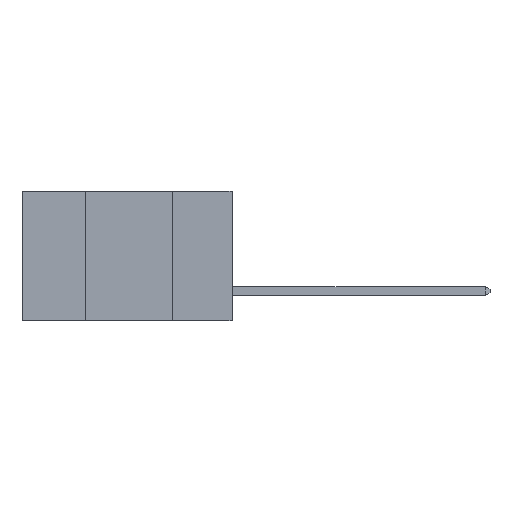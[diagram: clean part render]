
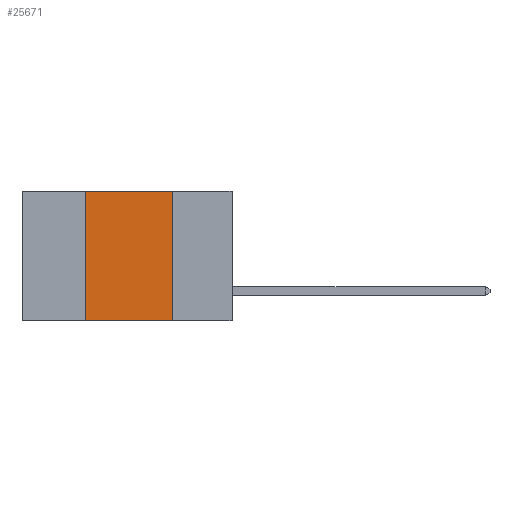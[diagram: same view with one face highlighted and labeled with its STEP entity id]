
A CAD part, left-side view. The second image highlights one B-rep face of the part: STEP entity #25671.
In plain terms, the highlighted planar face has unit normal (-1, 0, 0).
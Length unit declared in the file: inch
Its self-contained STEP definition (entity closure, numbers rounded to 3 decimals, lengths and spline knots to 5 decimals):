
#532 = VERTEX_POINT ( 'NONE', #34800 ) ;
#2224 = ORIENTED_EDGE ( 'NONE', *, *, #3149, .F. ) ;
#2685 = VERTEX_POINT ( 'NONE', #16816 ) ;
#2779 = DIRECTION ( 'NONE',  ( 0., 0., -1. ) ) ;
#3076 = LINE ( 'NONE', #16476, #35487 ) ;
#3149 = EDGE_CURVE ( 'NONE', #21279, #20346, #15940, .T. ) ;
#3304 = DIRECTION ( 'NONE',  ( 0., -1., 0. ) ) ;
#5337 = ORIENTED_EDGE ( 'NONE', *, *, #33064, .F. ) ;
#8743 = CARTESIAN_POINT ( 'NONE',  ( 0., 0.42, 0. ) ) ;
#14089 = ORIENTED_EDGE ( 'NONE', *, *, #38648, .F. ) ;
#15940 = LINE ( 'NONE', #41463, #35038 ) ;
#16476 = CARTESIAN_POINT ( 'NONE',  ( 0., 0.6, -0.37 ) ) ;
#16816 = CARTESIAN_POINT ( 'NONE',  ( 0., 0.42, 0. ) ) ;
#17154 = ORIENTED_EDGE ( 'NONE', *, *, #32216, .T. ) ;
#20110 = EDGE_LOOP ( 'NONE', ( #2224, #5337, #14089, #17154 ) ) ;
#20346 = VERTEX_POINT ( 'NONE', #21355 ) ;
#21279 = VERTEX_POINT ( 'NONE', #41705 ) ;
#21355 = CARTESIAN_POINT ( 'NONE',  ( 0., 0.17, -0.37 ) ) ;
#22315 = DIRECTION ( 'NONE',  ( 0., 0., -1. ) ) ;
#22366 = DIRECTION ( 'NONE',  ( 1., 0., 0. ) ) ;
#24945 = DIRECTION ( 'NONE',  ( 0., -1., 0. ) ) ;
#25671 = ADVANCED_FACE ( 'NONE', ( #34273 ), #41514, .F. ) ;
#27435 = LINE ( 'NONE', #37673, #34966 ) ;
#27769 = VECTOR ( 'NONE', #37753, 39.37008 ) ;
#28650 = CARTESIAN_POINT ( 'NONE',  ( 0., 0.6, 0. ) ) ;
#32216 = EDGE_CURVE ( 'NONE', #532, #20346, #3076, .T. ) ;
#33064 = EDGE_CURVE ( 'NONE', #2685, #21279, #27435, .T. ) ;
#34273 = FACE_OUTER_BOUND ( 'NONE', #20110, .T. ) ;
#34800 = CARTESIAN_POINT ( 'NONE',  ( 0., 0.42, -0.37 ) ) ;
#34966 = VECTOR ( 'NONE', #24945, 39.37008 ) ;
#35038 = VECTOR ( 'NONE', #22315, 39.37008 ) ;
#35487 = VECTOR ( 'NONE', #3304, 39.37008 ) ;
#36306 = LINE ( 'NONE', #8743, #27769 ) ;
#36754 = AXIS2_PLACEMENT_3D ( 'NONE', #28650, #22366, #2779 ) ;
#37673 = CARTESIAN_POINT ( 'NONE',  ( 0., 0.6, 0. ) ) ;
#37753 = DIRECTION ( 'NONE',  ( 0., 0., 1. ) ) ;
#38648 = EDGE_CURVE ( 'NONE', #532, #2685, #36306, .T. ) ;
#41463 = CARTESIAN_POINT ( 'NONE',  ( 0., 0.17, 0. ) ) ;
#41514 = PLANE ( 'NONE',  #36754 ) ;
#41705 = CARTESIAN_POINT ( 'NONE',  ( 0., 0.17, 0. ) ) ;
